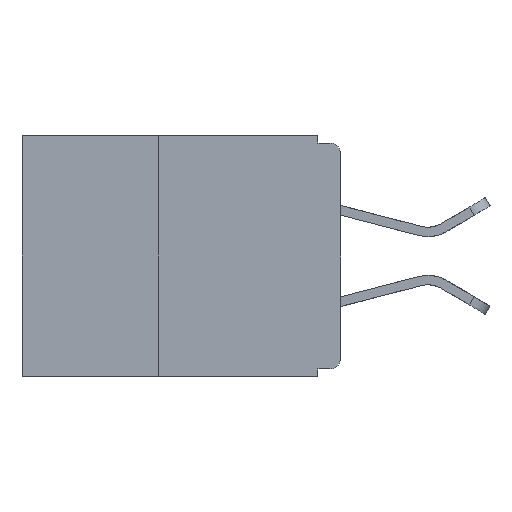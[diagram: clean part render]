
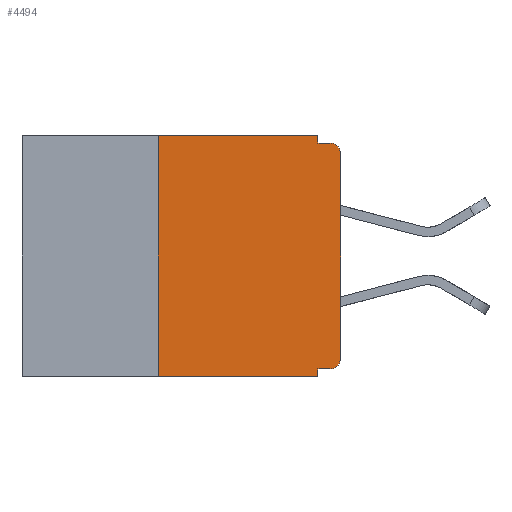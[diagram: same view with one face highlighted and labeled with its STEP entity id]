
A CAD part, left-side view. The second image highlights one B-rep face of the part: STEP entity #4494.
In plain terms, the highlighted planar face has unit normal (-1, 0, 0).
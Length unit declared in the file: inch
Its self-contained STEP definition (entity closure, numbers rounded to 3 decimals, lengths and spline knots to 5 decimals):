
#1 = AXIS2_PLACEMENT_3D ( 'NONE', #12068, #27291, #14258 ) ;
#167 = DIRECTION ( 'NONE',  ( 0., -1., 0. ) ) ;
#324 = CIRCLE ( 'NONE', #20422, 0.015 ) ;
#653 = ORIENTED_EDGE ( 'NONE', *, *, #28260, .F. ) ;
#669 = CARTESIAN_POINT ( 'NONE',  ( 0., 0.25, -0.33 ) ) ;
#735 = EDGE_CURVE ( 'NONE', #3746, #21966, #7305, .T. ) ;
#918 = EDGE_CURVE ( 'NONE', #7392, #23649, #26515, .T. ) ;
#1120 = LINE ( 'NONE', #22231, #24177 ) ;
#1710 = DIRECTION ( 'NONE',  ( -1., 0., 0. ) ) ;
#3229 = LINE ( 'NONE', #23690, #9989 ) ;
#3241 = ORIENTED_EDGE ( 'NONE', *, *, #918, .F. ) ;
#3746 = VERTEX_POINT ( 'NONE', #16643 ) ;
#3988 = DIRECTION ( 'NONE',  ( 0., 0., 1. ) ) ;
#4494 = ADVANCED_FACE ( 'NONE', ( #21446 ), #21650, .F. ) ;
#5611 = CARTESIAN_POINT ( 'NONE',  ( 0., 0., -0.32 ) ) ;
#6241 = VECTOR ( 'NONE', #18911, 39.37008 ) ;
#6404 = DIRECTION ( 'NONE',  ( 0., 0., 1. ) ) ;
#7025 = EDGE_CURVE ( 'NONE', #13582, #26866, #324, .T. ) ;
#7305 = CIRCLE ( 'NONE', #1, 0.015 ) ;
#7392 = VERTEX_POINT ( 'NONE', #9907 ) ;
#7593 = CARTESIAN_POINT ( 'NONE',  ( 0., 0.25, 0. ) ) ;
#8074 = VECTOR ( 'NONE', #167, 39.37008 ) ;
#8550 = CARTESIAN_POINT ( 'NONE',  ( 0., 0.437, 0. ) ) ;
#8643 = AXIS2_PLACEMENT_3D ( 'NONE', #8550, #10771, #26068 ) ;
#8675 = ORIENTED_EDGE ( 'NONE', *, *, #11510, .F. ) ;
#9001 = ORIENTED_EDGE ( 'NONE', *, *, #25395, .T. ) ;
#9907 = CARTESIAN_POINT ( 'NONE',  ( 0., 0.031, 0. ) ) ;
#9989 = VECTOR ( 'NONE', #10581, 39.37008 ) ;
#10469 = CARTESIAN_POINT ( 'NONE',  ( 0., 0.015, -0.01 ) ) ;
#10581 = DIRECTION ( 'NONE',  ( 0., 0., -1. ) ) ;
#10709 = ORIENTED_EDGE ( 'NONE', *, *, #26833, .F. ) ;
#10771 = DIRECTION ( 'NONE',  ( 1., 0., 0. ) ) ;
#10815 = LINE ( 'NONE', #16883, #26876 ) ;
#11510 = EDGE_CURVE ( 'NONE', #3746, #23396, #18652, .T. ) ;
#11911 = CARTESIAN_POINT ( 'NONE',  ( 0., 0., -0.305 ) ) ;
#12068 = CARTESIAN_POINT ( 'NONE',  ( 0., 0.015, -0.305 ) ) ;
#13543 = DIRECTION ( 'NONE',  ( 0., -1., 0. ) ) ;
#13582 = VERTEX_POINT ( 'NONE', #15099 ) ;
#13810 = CARTESIAN_POINT ( 'NONE',  ( 0., 0.437, -0.33 ) ) ;
#13959 = LINE ( 'NONE', #13810, #8074 ) ;
#14258 = DIRECTION ( 'NONE',  ( 0., 0., -1. ) ) ;
#14804 = ORIENTED_EDGE ( 'NONE', *, *, #7025, .T. ) ;
#15099 = CARTESIAN_POINT ( 'NONE',  ( 0., 0., -0.025 ) ) ;
#15215 = CARTESIAN_POINT ( 'NONE',  ( 0., 0.015, -0.025 ) ) ;
#16643 = CARTESIAN_POINT ( 'NONE',  ( 0., 0.015, -0.32 ) ) ;
#16883 = CARTESIAN_POINT ( 'NONE',  ( 0., 0.437, 0. ) ) ;
#17393 = CARTESIAN_POINT ( 'NONE',  ( 0., 0.25, -0.33 ) ) ;
#17413 = DIRECTION ( 'NONE',  ( 0., 0., -1. ) ) ;
#18652 = LINE ( 'NONE', #5611, #6241 ) ;
#18813 = EDGE_CURVE ( 'NONE', #23649, #26866, #1120, .T. ) ;
#18890 = VECTOR ( 'NONE', #6404, 39.37008 ) ;
#18907 = CARTESIAN_POINT ( 'NONE',  ( 0., 0.031, -0.01 ) ) ;
#18911 = DIRECTION ( 'NONE',  ( 0., 1., 0. ) ) ;
#19059 = DIRECTION ( 'NONE',  ( 0., -1., 0. ) ) ;
#19063 = VERTEX_POINT ( 'NONE', #669 ) ;
#19508 = CARTESIAN_POINT ( 'NONE',  ( 0., 0., 0. ) ) ;
#19592 = LINE ( 'NONE', #17393, #18890 ) ;
#20015 = VECTOR ( 'NONE', #27822, 39.37008 ) ;
#20422 = AXIS2_PLACEMENT_3D ( 'NONE', #15215, #1710, #17413 ) ;
#21395 = EDGE_LOOP ( 'NONE', ( #25065, #14804, #24730, #3241, #10709, #653, #9001, #24103, #8675, #26826 ) ) ;
#21446 = FACE_OUTER_BOUND ( 'NONE', #21395, .T. ) ;
#21650 = PLANE ( 'NONE',  #8643 ) ;
#21966 = VERTEX_POINT ( 'NONE', #11911 ) ;
#22231 = CARTESIAN_POINT ( 'NONE',  ( 0., 0., -0.01 ) ) ;
#22404 = CARTESIAN_POINT ( 'NONE',  ( 0., 0.031, -0.32 ) ) ;
#22490 = EDGE_CURVE ( 'NONE', #23396, #25828, #3229, .T. ) ;
#23396 = VERTEX_POINT ( 'NONE', #22404 ) ;
#23649 = VERTEX_POINT ( 'NONE', #18907 ) ;
#23690 = CARTESIAN_POINT ( 'NONE',  ( 0., 0.031, -0.33 ) ) ;
#24103 = ORIENTED_EDGE ( 'NONE', *, *, #22490, .F. ) ;
#24177 = VECTOR ( 'NONE', #13543, 39.37008 ) ;
#24456 = VECTOR ( 'NONE', #3988, 39.37008 ) ;
#24730 = ORIENTED_EDGE ( 'NONE', *, *, #18813, .F. ) ;
#25065 = ORIENTED_EDGE ( 'NONE', *, *, #27566, .T. ) ;
#25138 = LINE ( 'NONE', #19508, #24456 ) ;
#25395 = EDGE_CURVE ( 'NONE', #19063, #25828, #13959, .T. ) ;
#25701 = CARTESIAN_POINT ( 'NONE',  ( 0., 0.031, 0. ) ) ;
#25828 = VERTEX_POINT ( 'NONE', #28229 ) ;
#26068 = DIRECTION ( 'NONE',  ( 0., 0., -1. ) ) ;
#26515 = LINE ( 'NONE', #25701, #20015 ) ;
#26826 = ORIENTED_EDGE ( 'NONE', *, *, #735, .T. ) ;
#26833 = EDGE_CURVE ( 'NONE', #27923, #7392, #10815, .T. ) ;
#26866 = VERTEX_POINT ( 'NONE', #10469 ) ;
#26876 = VECTOR ( 'NONE', #19059, 39.37008 ) ;
#27291 = DIRECTION ( 'NONE',  ( -1., 0., 0. ) ) ;
#27566 = EDGE_CURVE ( 'NONE', #21966, #13582, #25138, .T. ) ;
#27822 = DIRECTION ( 'NONE',  ( 0., 0., -1. ) ) ;
#27923 = VERTEX_POINT ( 'NONE', #7593 ) ;
#28229 = CARTESIAN_POINT ( 'NONE',  ( 0., 0.031, -0.33 ) ) ;
#28260 = EDGE_CURVE ( 'NONE', #19063, #27923, #19592, .T. ) ;
